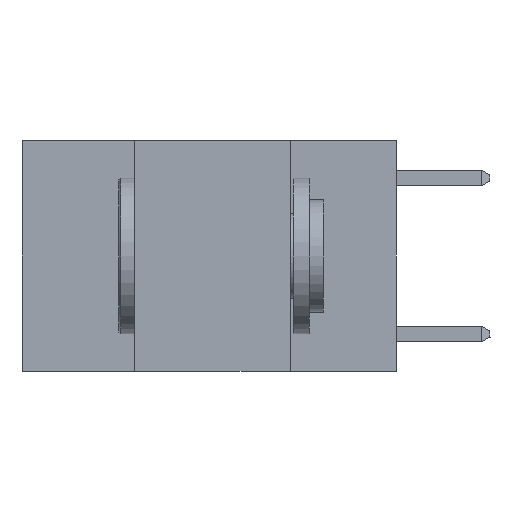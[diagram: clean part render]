
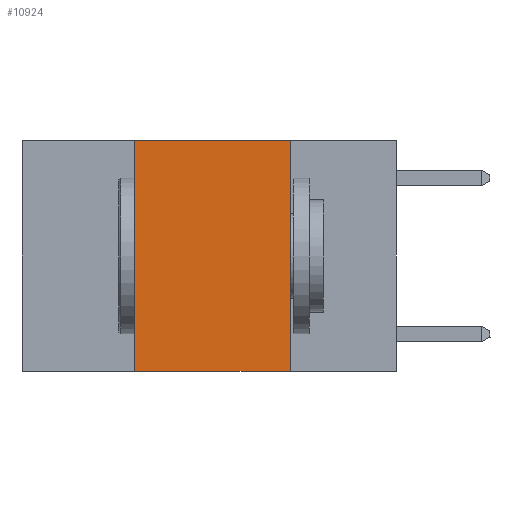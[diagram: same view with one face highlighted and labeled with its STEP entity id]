
A CAD part, left-side view. The second image highlights one B-rep face of the part: STEP entity #10924.
In plain terms, the highlighted planar face has unit normal (-1, 0, 0).
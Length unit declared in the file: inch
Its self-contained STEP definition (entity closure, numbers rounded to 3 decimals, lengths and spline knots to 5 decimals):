
#139 = DIRECTION ( 'NONE',  ( 0., 0., -1. ) ) ;
#367 = VERTEX_POINT ( 'NONE', #8325 ) ;
#821 = LINE ( 'NONE', #7493, #7751 ) ;
#871 = DIRECTION ( 'NONE',  ( 0., -1., 0. ) ) ;
#1468 = ORIENTED_EDGE ( 'NONE', *, *, #6096, .F. ) ;
#1935 = CARTESIAN_POINT ( 'NONE',  ( 0., 0.42, -0.37 ) ) ;
#3156 = CARTESIAN_POINT ( 'NONE',  ( 0., 0.17, -0.37 ) ) ;
#3772 = CARTESIAN_POINT ( 'NONE',  ( 0., 0.6, 0. ) ) ;
#4171 = ORIENTED_EDGE ( 'NONE', *, *, #6097, .F. ) ;
#4476 = ORIENTED_EDGE ( 'NONE', *, *, #6131, .T. ) ;
#4589 = FACE_OUTER_BOUND ( 'NONE', #5417, .T. ) ;
#4806 = CARTESIAN_POINT ( 'NONE',  ( 0., 0.42, 0. ) ) ;
#4839 = VECTOR ( 'NONE', #6683, 39.37008 ) ;
#5352 = VERTEX_POINT ( 'NONE', #1935 ) ;
#5417 = EDGE_LOOP ( 'NONE', ( #1468, #7435, #4171, #4476 ) ) ;
#5674 = EDGE_CURVE ( 'NONE', #8632, #367, #9574, .T. ) ;
#5702 = VECTOR ( 'NONE', #5735, 39.37008 ) ;
#5735 = DIRECTION ( 'NONE',  ( 0., 0., 1. ) ) ;
#6096 = EDGE_CURVE ( 'NONE', #367, #7365, #821, .T. ) ;
#6097 = EDGE_CURVE ( 'NONE', #5352, #8632, #8197, .T. ) ;
#6131 = EDGE_CURVE ( 'NONE', #5352, #7365, #7226, .T. ) ;
#6683 = DIRECTION ( 'NONE',  ( 0., -1., 0. ) ) ;
#6752 = CARTESIAN_POINT ( 'NONE',  ( 0., 0.42, 0. ) ) ;
#7226 = LINE ( 'NONE', #10476, #4839 ) ;
#7365 = VERTEX_POINT ( 'NONE', #3156 ) ;
#7398 = DIRECTION ( 'NONE',  ( 1., 0., 0. ) ) ;
#7435 = ORIENTED_EDGE ( 'NONE', *, *, #5674, .F. ) ;
#7493 = CARTESIAN_POINT ( 'NONE',  ( 0., 0.17, 0. ) ) ;
#7751 = VECTOR ( 'NONE', #9684, 39.37008 ) ;
#8197 = LINE ( 'NONE', #4806, #5702 ) ;
#8325 = CARTESIAN_POINT ( 'NONE',  ( 0., 0.17, 0. ) ) ;
#8632 = VERTEX_POINT ( 'NONE', #6752 ) ;
#9341 = VECTOR ( 'NONE', #871, 39.37008 ) ;
#9574 = LINE ( 'NONE', #10944, #9341 ) ;
#9684 = DIRECTION ( 'NONE',  ( 0., 0., -1. ) ) ;
#10362 = PLANE ( 'NONE',  #10493 ) ;
#10476 = CARTESIAN_POINT ( 'NONE',  ( 0., 0.6, -0.37 ) ) ;
#10493 = AXIS2_PLACEMENT_3D ( 'NONE', #3772, #7398, #139 ) ;
#10924 = ADVANCED_FACE ( 'NONE', ( #4589 ), #10362, .F. ) ;
#10944 = CARTESIAN_POINT ( 'NONE',  ( 0., 0.6, 0. ) ) ;
